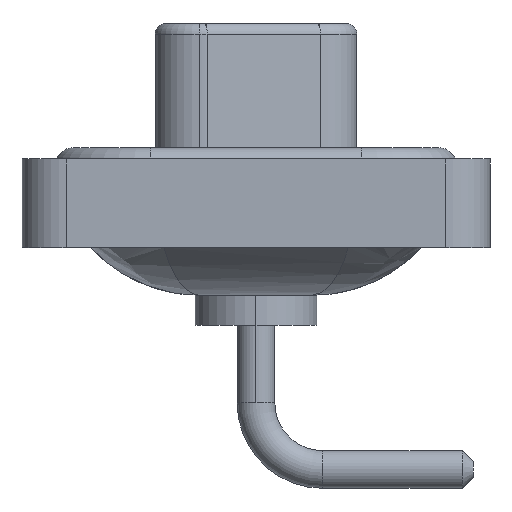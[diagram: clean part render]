
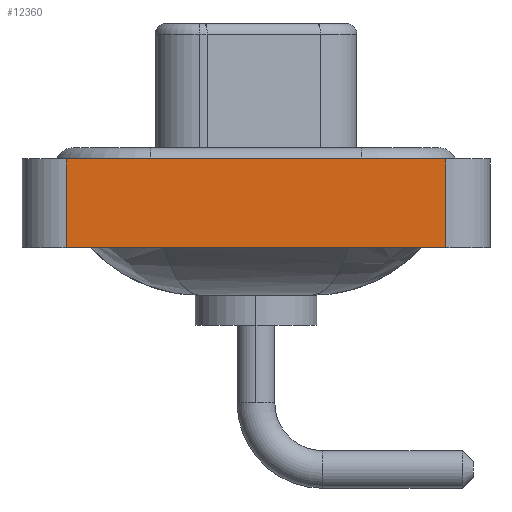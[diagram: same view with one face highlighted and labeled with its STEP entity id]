
A CAD part, left-side view. The second image highlights one B-rep face of the part: STEP entity #12360.
In plain terms, the highlighted planar face has unit normal (-1, 0, 0).
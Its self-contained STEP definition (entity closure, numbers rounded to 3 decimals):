
#274 = CARTESIAN_POINT ( 'NONE',  ( -7.35, -8.55, -3.6 ) ) ;
#389 = DIRECTION ( 'NONE',  ( 0., 0., 1. ) ) ;
#592 = AXIS2_PLACEMENT_3D ( 'NONE', #9288, #3816, #4906 ) ;
#1059 = FACE_OUTER_BOUND ( 'NONE', #1752, .T. ) ;
#1752 = EDGE_LOOP ( 'NONE', ( #16079, #10475, #10754, #13520 ) ) ;
#1923 = CARTESIAN_POINT ( 'NONE',  ( -7.35, -8.55, -3.6 ) ) ;
#2511 = DIRECTION ( 'NONE',  ( 0., -1., 0. ) ) ;
#3469 = VECTOR ( 'NONE', #7391, 1000. ) ;
#3816 = DIRECTION ( 'NONE',  ( -1., 0., 0. ) ) ;
#4597 = CARTESIAN_POINT ( 'NONE',  ( -7.35, 8.55, 0.4 ) ) ;
#4906 = DIRECTION ( 'NONE',  ( 0., 0., 1. ) ) ;
#5020 = VECTOR ( 'NONE', #14528, 1000. ) ;
#5527 = CARTESIAN_POINT ( 'NONE',  ( -7.35, 8.55, -3.6 ) ) ;
#5953 = VERTEX_POINT ( 'NONE', #5527 ) ;
#6228 = CARTESIAN_POINT ( 'NONE',  ( -7.35, 8.55, -3.6 ) ) ;
#7206 = CARTESIAN_POINT ( 'NONE',  ( -7.35, -8.55, -3.6 ) ) ;
#7391 = DIRECTION ( 'NONE',  ( 0., -1., 0. ) ) ;
#7909 = PLANE ( 'NONE',  #592 ) ;
#8160 = VERTEX_POINT ( 'NONE', #4597 ) ;
#9008 = VECTOR ( 'NONE', #389, 1000. ) ;
#9288 = CARTESIAN_POINT ( 'NONE',  ( -7.35, -8.55, -3.6 ) ) ;
#10388 = LINE ( 'NONE', #7206, #5020 ) ;
#10475 = ORIENTED_EDGE ( 'NONE', *, *, #13159, .F. ) ;
#10718 = CARTESIAN_POINT ( 'NONE',  ( -7.35, -8.55, 0.4 ) ) ;
#10754 = ORIENTED_EDGE ( 'NONE', *, *, #11810, .F. ) ;
#11178 = VECTOR ( 'NONE', #2511, 1000. ) ;
#11556 = VERTEX_POINT ( 'NONE', #16777 ) ;
#11810 = EDGE_CURVE ( 'NONE', #5953, #8160, #13209, .T. ) ;
#12213 = LINE ( 'NONE', #10718, #11178 ) ;
#12360 = ADVANCED_FACE ( 'NONE', ( #1059 ), #7909, .T. ) ;
#13159 = EDGE_CURVE ( 'NONE', #8160, #11556, #12213, .T. ) ;
#13209 = LINE ( 'NONE', #6228, #9008 ) ;
#13419 = LINE ( 'NONE', #1923, #3469 ) ;
#13520 = ORIENTED_EDGE ( 'NONE', *, *, #15898, .T. ) ;
#14528 = DIRECTION ( 'NONE',  ( 0., 0., 1. ) ) ;
#15898 = EDGE_CURVE ( 'NONE', #5953, #17127, #13419, .T. ) ;
#16079 = ORIENTED_EDGE ( 'NONE', *, *, #17818, .T. ) ;
#16777 = CARTESIAN_POINT ( 'NONE',  ( -7.35, -8.55, 0.4 ) ) ;
#17127 = VERTEX_POINT ( 'NONE', #274 ) ;
#17818 = EDGE_CURVE ( 'NONE', #17127, #11556, #10388, .T. ) ;
